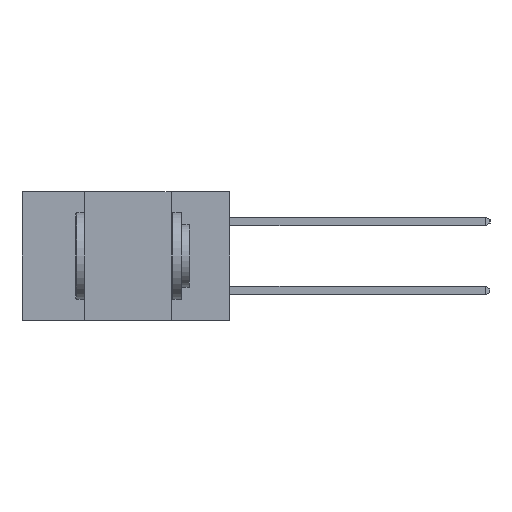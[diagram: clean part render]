
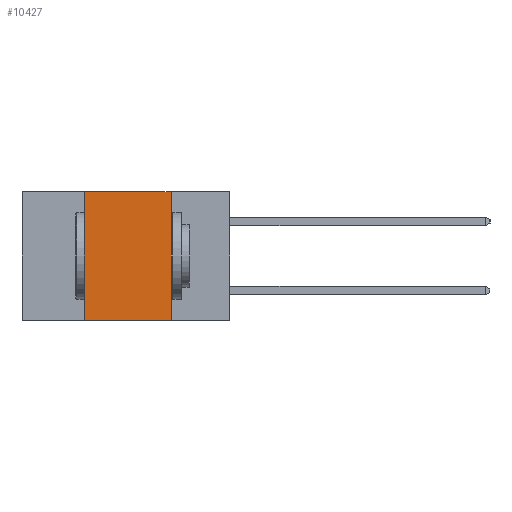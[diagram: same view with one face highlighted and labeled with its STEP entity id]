
A CAD part, left-side view. The second image highlights one B-rep face of the part: STEP entity #10427.
In plain terms, the highlighted planar face has unit normal (-1, 0, 0).
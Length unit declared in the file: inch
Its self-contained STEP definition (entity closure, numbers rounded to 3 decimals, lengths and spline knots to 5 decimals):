
#38 = CARTESIAN_POINT ( 'NONE',  ( 0., 0.42, -0.37 ) ) ;
#297 = VECTOR ( 'NONE', #749, 39.37008 ) ;
#749 = DIRECTION ( 'NONE',  ( 0., 0., -1. ) ) ;
#760 = EDGE_CURVE ( 'NONE', #5577, #4620, #15388, .T. ) ;
#955 = VECTOR ( 'NONE', #14818, 39.37008 ) ;
#2519 = CARTESIAN_POINT ( 'NONE',  ( 0., 0.42, 0. ) ) ;
#3453 = ORIENTED_EDGE ( 'NONE', *, *, #13495, .F. ) ;
#4620 = VERTEX_POINT ( 'NONE', #21756 ) ;
#5446 = LINE ( 'NONE', #6288, #955 ) ;
#5577 = VERTEX_POINT ( 'NONE', #38 ) ;
#5791 = EDGE_LOOP ( 'NONE', ( #21190, #3453, #8545, #13065 ) ) ;
#5805 = CARTESIAN_POINT ( 'NONE',  ( 0., 0.42, 0. ) ) ;
#6288 = CARTESIAN_POINT ( 'NONE',  ( 0., 0.6, 0. ) ) ;
#6291 = VECTOR ( 'NONE', #19544, 39.37008 ) ;
#6774 = PLANE ( 'NONE',  #13900 ) ;
#7215 = CARTESIAN_POINT ( 'NONE',  ( 0., 0.17, 0. ) ) ;
#7525 = DIRECTION ( 'NONE',  ( 0., 0., 1. ) ) ;
#8545 = ORIENTED_EDGE ( 'NONE', *, *, #17191, .F. ) ;
#8592 = CARTESIAN_POINT ( 'NONE',  ( 0., 0.6, 0. ) ) ;
#8714 = EDGE_CURVE ( 'NONE', #19181, #4620, #8834, .T. ) ;
#8834 = LINE ( 'NONE', #14384, #297 ) ;
#9427 = VERTEX_POINT ( 'NONE', #2519 ) ;
#9823 = FACE_OUTER_BOUND ( 'NONE', #5791, .T. ) ;
#10317 = DIRECTION ( 'NONE',  ( 0., 0., -1. ) ) ;
#10427 = ADVANCED_FACE ( 'NONE', ( #9823 ), #6774, .F. ) ;
#12773 = VECTOR ( 'NONE', #7525, 39.37008 ) ;
#13065 = ORIENTED_EDGE ( 'NONE', *, *, #760, .T. ) ;
#13314 = LINE ( 'NONE', #5805, #12773 ) ;
#13495 = EDGE_CURVE ( 'NONE', #9427, #19181, #5446, .T. ) ;
#13900 = AXIS2_PLACEMENT_3D ( 'NONE', #8592, #20618, #10317 ) ;
#14384 = CARTESIAN_POINT ( 'NONE',  ( 0., 0.17, 0. ) ) ;
#14788 = CARTESIAN_POINT ( 'NONE',  ( 0., 0.6, -0.37 ) ) ;
#14818 = DIRECTION ( 'NONE',  ( 0., -1., 0. ) ) ;
#15388 = LINE ( 'NONE', #14788, #6291 ) ;
#17191 = EDGE_CURVE ( 'NONE', #5577, #9427, #13314, .T. ) ;
#19181 = VERTEX_POINT ( 'NONE', #7215 ) ;
#19544 = DIRECTION ( 'NONE',  ( 0., -1., 0. ) ) ;
#20618 = DIRECTION ( 'NONE',  ( 1., 0., 0. ) ) ;
#21190 = ORIENTED_EDGE ( 'NONE', *, *, #8714, .F. ) ;
#21756 = CARTESIAN_POINT ( 'NONE',  ( 0., 0.17, -0.37 ) ) ;
